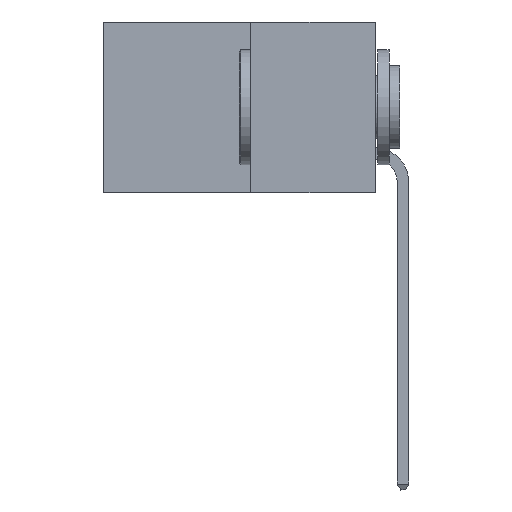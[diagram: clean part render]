
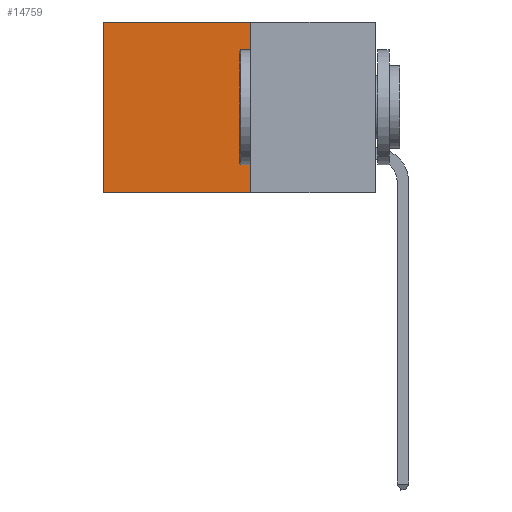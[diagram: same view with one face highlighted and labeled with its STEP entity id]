
A CAD part, left-side view. The second image highlights one B-rep face of the part: STEP entity #14759.
In plain terms, the highlighted planar face has unit normal (-1, 0, 0).
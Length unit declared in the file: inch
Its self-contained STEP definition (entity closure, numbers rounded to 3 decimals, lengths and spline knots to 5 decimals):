
#893 = VECTOR ( 'NONE', #9979, 39.37008 ) ;
#1009 = CARTESIAN_POINT ( 'NONE',  ( 0.277, 0.27, 0. ) ) ;
#1117 = LINE ( 'NONE', #11389, #13170 ) ;
#1254 = CARTESIAN_POINT ( 'NONE',  ( 0.277, 0.27, -0.37 ) ) ;
#1921 = VERTEX_POINT ( 'NONE', #11750 ) ;
#3229 = PLANE ( 'NONE',  #7111 ) ;
#4007 = CARTESIAN_POINT ( 'NONE',  ( 0.277, 0.59, -0.37 ) ) ;
#4570 = ORIENTED_EDGE ( 'NONE', *, *, #12717, .F. ) ;
#5726 = DIRECTION ( 'NONE',  ( 1., 0., 0. ) ) ;
#6025 = EDGE_CURVE ( 'NONE', #1921, #9491, #7186, .T. ) ;
#6597 = CARTESIAN_POINT ( 'NONE',  ( 0.277, 0.59, -0.37 ) ) ;
#7032 = DIRECTION ( 'NONE',  ( 0., 1., 0. ) ) ;
#7111 = AXIS2_PLACEMENT_3D ( 'NONE', #11507, #5726, #13693 ) ;
#7186 = LINE ( 'NONE', #1254, #9933 ) ;
#7432 = ORIENTED_EDGE ( 'NONE', *, *, #7522, .T. ) ;
#7522 = EDGE_CURVE ( 'NONE', #13796, #9491, #10412, .T. ) ;
#7825 = ORIENTED_EDGE ( 'NONE', *, *, #8508, .T. ) ;
#8011 = DIRECTION ( 'NONE',  ( 0., 0., -1. ) ) ;
#8235 = VECTOR ( 'NONE', #7032, 39.37008 ) ;
#8508 = EDGE_CURVE ( 'NONE', #12931, #13796, #8582, .T. ) ;
#8582 = LINE ( 'NONE', #1009, #8235 ) ;
#9491 = VERTEX_POINT ( 'NONE', #6597 ) ;
#9933 = VECTOR ( 'NONE', #10696, 39.37008 ) ;
#9979 = DIRECTION ( 'NONE',  ( 0., 0., -1. ) ) ;
#10412 = LINE ( 'NONE', #4007, #893 ) ;
#10446 = CARTESIAN_POINT ( 'NONE',  ( 0.277, 0.59, 0. ) ) ;
#10510 = ORIENTED_EDGE ( 'NONE', *, *, #6025, .F. ) ;
#10696 = DIRECTION ( 'NONE',  ( 0., 1., 0. ) ) ;
#10733 = FACE_OUTER_BOUND ( 'NONE', #13393, .T. ) ;
#11389 = CARTESIAN_POINT ( 'NONE',  ( 0.277, 0.27, -0.37 ) ) ;
#11507 = CARTESIAN_POINT ( 'NONE',  ( 0.277, 0.27, -0.37 ) ) ;
#11750 = CARTESIAN_POINT ( 'NONE',  ( 0.277, 0.27, -0.37 ) ) ;
#12717 = EDGE_CURVE ( 'NONE', #12931, #1921, #1117, .T. ) ;
#12931 = VERTEX_POINT ( 'NONE', #13187 ) ;
#13170 = VECTOR ( 'NONE', #8011, 39.37008 ) ;
#13187 = CARTESIAN_POINT ( 'NONE',  ( 0.277, 0.27, 0. ) ) ;
#13393 = EDGE_LOOP ( 'NONE', ( #7432, #10510, #4570, #7825 ) ) ;
#13693 = DIRECTION ( 'NONE',  ( 0., 0., -1. ) ) ;
#13796 = VERTEX_POINT ( 'NONE', #10446 ) ;
#14759 = ADVANCED_FACE ( 'NONE', ( #10733 ), #3229, .F. ) ;
